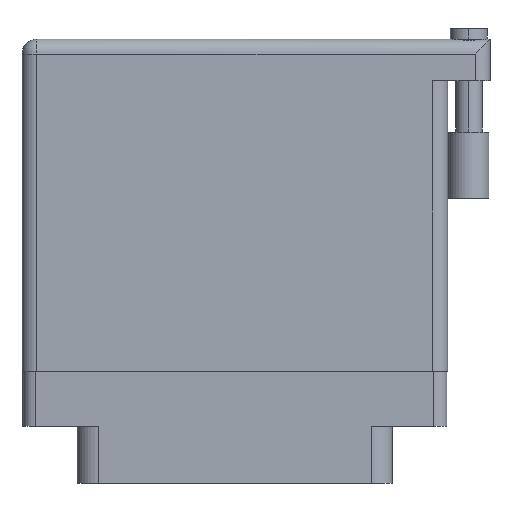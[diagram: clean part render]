
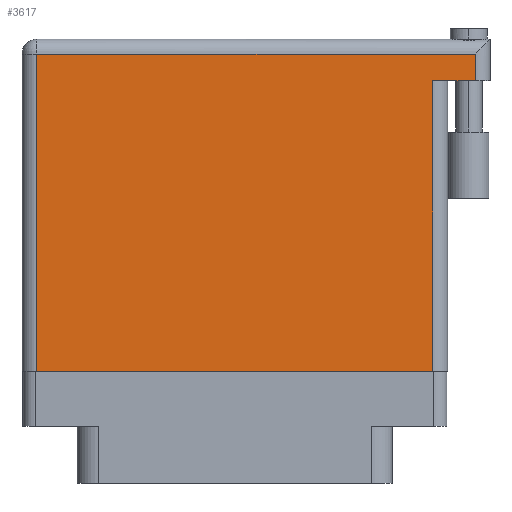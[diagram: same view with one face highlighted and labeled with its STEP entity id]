
A CAD part, front view. The second image highlights one B-rep face of the part: STEP entity #3617.
In plain terms, the highlighted face is planar.
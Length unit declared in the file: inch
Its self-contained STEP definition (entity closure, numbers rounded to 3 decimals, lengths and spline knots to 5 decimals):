
#270 = VECTOR ( 'NONE', #14919, 39.37008 ) ;
#643 = LINE ( 'NONE', #33043, #21640 ) ;
#649 = EDGE_CURVE ( 'NONE', #33495, #10713, #32149, .T. ) ;
#1023 = EDGE_CURVE ( 'NONE', #33876, #10713, #19851, .T. ) ;
#1668 = VERTEX_POINT ( 'NONE', #13473 ) ;
#3617 = ADVANCED_FACE ( 'NONE', ( #10423 ), #31973, .F. ) ;
#4635 = CARTESIAN_POINT ( 'NONE',  ( 2.138, 1.369, 0. ) ) ;
#5760 = DIRECTION ( 'NONE',  ( -1., 0., 0. ) ) ;
#6146 = AXIS2_PLACEMENT_3D ( 'NONE', #13564, #24107, #7980 ) ;
#6626 = LINE ( 'NONE', #14671, #15176 ) ;
#7980 = DIRECTION ( 'NONE',  ( -1., 0., 0. ) ) ;
#8391 = CARTESIAN_POINT ( 'NONE',  ( 0., 1.496, 0. ) ) ;
#8792 = ORIENTED_EDGE ( 'NONE', *, *, #11446, .T. ) ;
#8954 = ORIENTED_EDGE ( 'NONE', *, *, #12200, .T. ) ;
#10423 = FACE_OUTER_BOUND ( 'NONE', #26709, .T. ) ;
#10488 = ORIENTED_EDGE ( 'NONE', *, *, #32245, .T. ) ;
#10713 = VERTEX_POINT ( 'NONE', #21189 ) ;
#10773 = DIRECTION ( 'NONE',  ( 0., 1., 0. ) ) ;
#11446 = EDGE_CURVE ( 'NONE', #30419, #17886, #23336, .T. ) ;
#12200 = EDGE_CURVE ( 'NONE', #1668, #30419, #19758, .T. ) ;
#13473 = CARTESIAN_POINT ( 'NONE',  ( 2.138, 1.496, 0. ) ) ;
#13564 = CARTESIAN_POINT ( 'NONE',  ( 0., 1.566, 0. ) ) ;
#14671 = CARTESIAN_POINT ( 'NONE',  ( 2.138, 1.566, 0. ) ) ;
#14919 = DIRECTION ( 'NONE',  ( -1., 0., 0. ) ) ;
#15176 = VECTOR ( 'NONE', #25365, 39.37008 ) ;
#15463 = VECTOR ( 'NONE', #19877, 39.37008 ) ;
#15716 = CARTESIAN_POINT ( 'NONE',  ( 1.938, 0., 0. ) ) ;
#16231 = ORIENTED_EDGE ( 'NONE', *, *, #649, .T. ) ;
#17418 = ORIENTED_EDGE ( 'NONE', *, *, #18881, .T. ) ;
#17886 = VERTEX_POINT ( 'NONE', #31991 ) ;
#18881 = EDGE_CURVE ( 'NONE', #33876, #1668, #6626, .T. ) ;
#19758 = LINE ( 'NONE', #8391, #30106 ) ;
#19851 = LINE ( 'NONE', #21071, #270 ) ;
#19877 = DIRECTION ( 'NONE',  ( 0., -1., 0. ) ) ;
#21071 = CARTESIAN_POINT ( 'NONE',  ( 2.208, 1.369, 0. ) ) ;
#21189 = CARTESIAN_POINT ( 'NONE',  ( 1.938, 1.369, 0. ) ) ;
#21640 = VECTOR ( 'NONE', #24999, 39.37008 ) ;
#22775 = VECTOR ( 'NONE', #10773, 39.37008 ) ;
#23336 = LINE ( 'NONE', #34005, #15463 ) ;
#24107 = DIRECTION ( 'NONE',  ( 0., 0., -1. ) ) ;
#24344 = CARTESIAN_POINT ( 'NONE',  ( 0.07, 1.496, 0. ) ) ;
#24999 = DIRECTION ( 'NONE',  ( 1., 0., 0. ) ) ;
#25365 = DIRECTION ( 'NONE',  ( 0., 1., 0. ) ) ;
#26709 = EDGE_LOOP ( 'NONE', ( #10488, #16231, #31129, #17418, #8954, #8792 ) ) ;
#26918 = CARTESIAN_POINT ( 'NONE',  ( 1.938, 1.369, 0. ) ) ;
#30106 = VECTOR ( 'NONE', #5760, 39.37008 ) ;
#30419 = VERTEX_POINT ( 'NONE', #24344 ) ;
#31129 = ORIENTED_EDGE ( 'NONE', *, *, #1023, .F. ) ;
#31973 = PLANE ( 'NONE',  #6146 ) ;
#31991 = CARTESIAN_POINT ( 'NONE',  ( 0.07, 0., 0. ) ) ;
#32149 = LINE ( 'NONE', #26918, #22775 ) ;
#32245 = EDGE_CURVE ( 'NONE', #17886, #33495, #643, .T. ) ;
#33043 = CARTESIAN_POINT ( 'NONE',  ( 0., 0., 0. ) ) ;
#33495 = VERTEX_POINT ( 'NONE', #15716 ) ;
#33876 = VERTEX_POINT ( 'NONE', #4635 ) ;
#34005 = CARTESIAN_POINT ( 'NONE',  ( 0.07, 0., 0. ) ) ;
